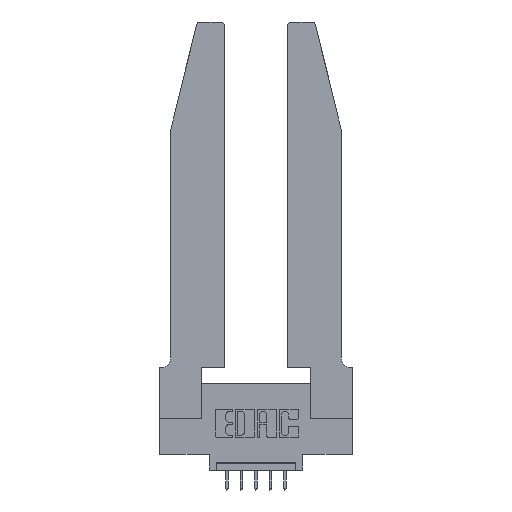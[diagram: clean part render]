
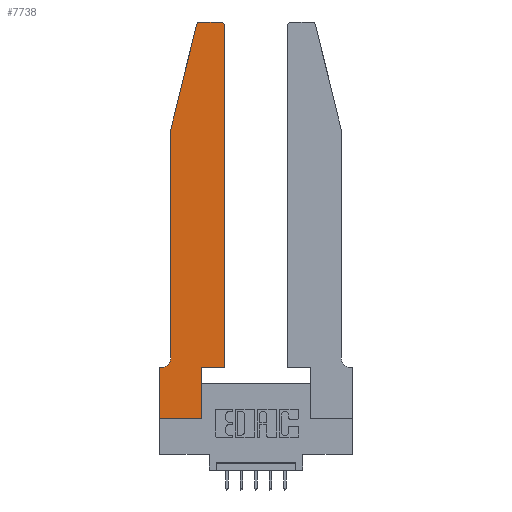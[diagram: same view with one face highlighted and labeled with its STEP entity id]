
A CAD part, top view. The second image highlights one B-rep face of the part: STEP entity #7738.
In plain terms, the highlighted planar face has unit normal (0, 0, 1).
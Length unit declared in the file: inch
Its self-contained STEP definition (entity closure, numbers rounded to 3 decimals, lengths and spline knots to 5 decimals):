
#335 = DIRECTION ( 'NONE',  ( 0., 0., 1. ) ) ;
#342 = VECTOR ( 'NONE', #3186, 39.37008 ) ;
#669 = DIRECTION ( 'NONE',  ( 1., 0., 0. ) ) ;
#903 = VERTEX_POINT ( 'NONE', #3557 ) ;
#917 = EDGE_LOOP ( 'NONE', ( #12621, #952, #5029, #2831, #6538, #11833, #9328, #13128, #4630, #1027, #4087, #11568 ) ) ;
#934 = CARTESIAN_POINT ( 'NONE',  ( 0.2865, 0.35, 0.37 ) ) ;
#952 = ORIENTED_EDGE ( 'NONE', *, *, #6176, .T. ) ;
#1027 = ORIENTED_EDGE ( 'NONE', *, *, #11764, .T. ) ;
#1371 = CARTESIAN_POINT ( 'NONE',  ( 0.4505, 0.35, 0.37 ) ) ;
#1515 = PLANE ( 'NONE',  #2457 ) ;
#1556 = CARTESIAN_POINT ( 'NONE',  ( 0.2865, 0., 0.37 ) ) ;
#1720 = FACE_OUTER_BOUND ( 'NONE', #917, .T. ) ;
#1979 = CARTESIAN_POINT ( 'NONE',  ( 0.4505, 0.35, 0.37 ) ) ;
#2457 = AXIS2_PLACEMENT_3D ( 'NONE', #9827, #335, #8782 ) ;
#2720 = VERTEX_POINT ( 'NONE', #11738 ) ;
#2820 = VERTEX_POINT ( 'NONE', #6566 ) ;
#2831 = ORIENTED_EDGE ( 'NONE', *, *, #12028, .T. ) ;
#3186 = DIRECTION ( 'NONE',  ( 0., 1., 0. ) ) ;
#3373 = DIRECTION ( 'NONE',  ( 1., 0., 0. ) ) ;
#3440 = DIRECTION ( 'NONE',  ( 0., -1., 0. ) ) ;
#3557 = CARTESIAN_POINT ( 'NONE',  ( 0.284, 2.75, 0.37 ) ) ;
#3901 = CARTESIAN_POINT ( 'NONE',  ( 0.4205, 2.72, 0.37 ) ) ;
#4087 = ORIENTED_EDGE ( 'NONE', *, *, #11320, .T. ) ;
#4164 = DIRECTION ( 'NONE',  ( -1., 0., 0. ) ) ;
#4184 = CARTESIAN_POINT ( 'NONE',  ( 0.25487, 2.72718, 0.37 ) ) ;
#4198 = CIRCLE ( 'NONE', #5496, 0.07 ) ;
#4211 = DIRECTION ( 'NONE',  ( 1., 0., 0. ) ) ;
#4247 = LINE ( 'NONE', #934, #342 ) ;
#4440 = VECTOR ( 'NONE', #10663, 39.37008 ) ;
#4483 = LINE ( 'NONE', #8693, #13086 ) ;
#4619 = CARTESIAN_POINT ( 'NONE',  ( 0.0755, 2., 0.37 ) ) ;
#4630 = ORIENTED_EDGE ( 'NONE', *, *, #9971, .T. ) ;
#4825 = CARTESIAN_POINT ( 'NONE',  ( 0.0755, 2., 0.37 ) ) ;
#4853 = CARTESIAN_POINT ( 'NONE',  ( 0., 0., 0.37 ) ) ;
#5012 = VERTEX_POINT ( 'NONE', #10673 ) ;
#5029 = ORIENTED_EDGE ( 'NONE', *, *, #6588, .T. ) ;
#5031 = VERTEX_POINT ( 'NONE', #8708 ) ;
#5044 = VERTEX_POINT ( 'NONE', #5320 ) ;
#5252 = AXIS2_PLACEMENT_3D ( 'NONE', #3901, #6189, #669 ) ;
#5320 = CARTESIAN_POINT ( 'NONE',  ( 0.0755, 0.42, 0.37 ) ) ;
#5329 = CARTESIAN_POINT ( 'NONE',  ( 0., 0., 0.37 ) ) ;
#5387 = LINE ( 'NONE', #5329, #11307 ) ;
#5454 = EDGE_CURVE ( 'NONE', #5761, #13148, #4483, .T. ) ;
#5496 = AXIS2_PLACEMENT_3D ( 'NONE', #6233, #9429, #4164 ) ;
#5695 = LINE ( 'NONE', #4619, #7223 ) ;
#5747 = CARTESIAN_POINT ( 'NONE',  ( 0.0755, 2., 0.37 ) ) ;
#5761 = VERTEX_POINT ( 'NONE', #4853 ) ;
#5821 = DIRECTION ( 'NONE',  ( 0., 1., 0. ) ) ;
#6176 = EDGE_CURVE ( 'NONE', #903, #11343, #12656, .T. ) ;
#6189 = DIRECTION ( 'NONE',  ( 0., 0., 1. ) ) ;
#6233 = CARTESIAN_POINT ( 'NONE',  ( 0.0055, 0.42, 0.37 ) ) ;
#6269 = CARTESIAN_POINT ( 'NONE',  ( 0.0755, 0.35, 0.37 ) ) ;
#6538 = ORIENTED_EDGE ( 'NONE', *, *, #6771, .T. ) ;
#6566 = CARTESIAN_POINT ( 'NONE',  ( 0.0055, 0.35, 0.37 ) ) ;
#6588 = EDGE_CURVE ( 'NONE', #11343, #10926, #8105, .T. ) ;
#6771 = EDGE_CURVE ( 'NONE', #5044, #2820, #4198, .T. ) ;
#6951 = CARTESIAN_POINT ( 'NONE',  ( 0.4505, 0.35, 0.37 ) ) ;
#7223 = VECTOR ( 'NONE', #7513, 39.37008 ) ;
#7232 = VERTEX_POINT ( 'NONE', #8052 ) ;
#7512 = VECTOR ( 'NONE', #10724, 39.37008 ) ;
#7513 = DIRECTION ( 'NONE',  ( 0., -1., 0. ) ) ;
#7565 = EDGE_CURVE ( 'NONE', #5031, #5761, #5387, .T. ) ;
#7738 = ADVANCED_FACE ( 'NONE', ( #1720 ), #1515, .T. ) ;
#7851 = EDGE_CURVE ( 'NONE', #5012, #903, #12698, .T. ) ;
#7936 = EDGE_CURVE ( 'NONE', #2820, #5031, #11850, .T. ) ;
#8052 = CARTESIAN_POINT ( 'NONE',  ( 0.4505, 2.72, 0.37 ) ) ;
#8105 = LINE ( 'NONE', #5747, #13288 ) ;
#8693 = CARTESIAN_POINT ( 'NONE',  ( 0., 0., 0.37 ) ) ;
#8708 = CARTESIAN_POINT ( 'NONE',  ( 0., 0.35, 0.37 ) ) ;
#8782 = DIRECTION ( 'NONE',  ( 1., 0., 0. ) ) ;
#9016 = DIRECTION ( 'NONE',  ( -0.239, -0.971, 0. ) ) ;
#9328 = ORIENTED_EDGE ( 'NONE', *, *, #7565, .T. ) ;
#9429 = DIRECTION ( 'NONE',  ( 0., 0., -1. ) ) ;
#9678 = CIRCLE ( 'NONE', #5252, 0.03 ) ;
#9827 = CARTESIAN_POINT ( 'NONE',  ( 0., 0.35, 0.37 ) ) ;
#9971 = EDGE_CURVE ( 'NONE', #13148, #2720, #4247, .T. ) ;
#10663 = DIRECTION ( 'NONE',  ( -1., 0., 0. ) ) ;
#10673 = CARTESIAN_POINT ( 'NONE',  ( 0.4205, 2.75, 0.37 ) ) ;
#10724 = DIRECTION ( 'NONE',  ( -1., 0., 0. ) ) ;
#10926 = VERTEX_POINT ( 'NONE', #4825 ) ;
#11006 = LINE ( 'NONE', #1371, #12540 ) ;
#11307 = VECTOR ( 'NONE', #3440, 39.37008 ) ;
#11320 = EDGE_CURVE ( 'NONE', #13415, #7232, #12457, .T. ) ;
#11321 = AXIS2_PLACEMENT_3D ( 'NONE', #13661, #11431, #4211 ) ;
#11343 = VERTEX_POINT ( 'NONE', #4184 ) ;
#11431 = DIRECTION ( 'NONE',  ( 0., 0., 1. ) ) ;
#11568 = ORIENTED_EDGE ( 'NONE', *, *, #13718, .T. ) ;
#11738 = CARTESIAN_POINT ( 'NONE',  ( 0.2865, 0.35, 0.37 ) ) ;
#11764 = EDGE_CURVE ( 'NONE', #2720, #13415, #11006, .T. ) ;
#11833 = ORIENTED_EDGE ( 'NONE', *, *, #7936, .T. ) ;
#11850 = LINE ( 'NONE', #6269, #7512 ) ;
#12028 = EDGE_CURVE ( 'NONE', #10926, #5044, #5695, .T. ) ;
#12351 = VECTOR ( 'NONE', #5821, 39.37008 ) ;
#12457 = LINE ( 'NONE', #6951, #12351 ) ;
#12540 = VECTOR ( 'NONE', #3373, 39.37008 ) ;
#12621 = ORIENTED_EDGE ( 'NONE', *, *, #7851, .T. ) ;
#12656 = CIRCLE ( 'NONE', #11321, 0.03 ) ;
#12698 = LINE ( 'NONE', #12899, #4440 ) ;
#12899 = CARTESIAN_POINT ( 'NONE',  ( 0.2605, 2.75, 0.37 ) ) ;
#12954 = DIRECTION ( 'NONE',  ( 1., 0., 0. ) ) ;
#13086 = VECTOR ( 'NONE', #12954, 39.37008 ) ;
#13128 = ORIENTED_EDGE ( 'NONE', *, *, #5454, .T. ) ;
#13148 = VERTEX_POINT ( 'NONE', #1556 ) ;
#13288 = VECTOR ( 'NONE', #9016, 39.37008 ) ;
#13415 = VERTEX_POINT ( 'NONE', #1979 ) ;
#13661 = CARTESIAN_POINT ( 'NONE',  ( 0.284, 2.72, 0.37 ) ) ;
#13718 = EDGE_CURVE ( 'NONE', #7232, #5012, #9678, .T. ) ;
